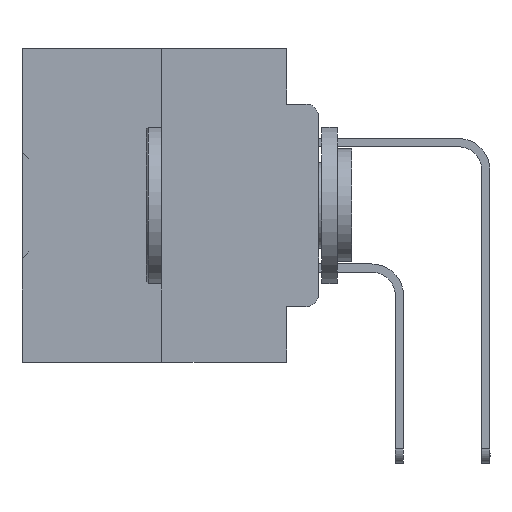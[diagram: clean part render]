
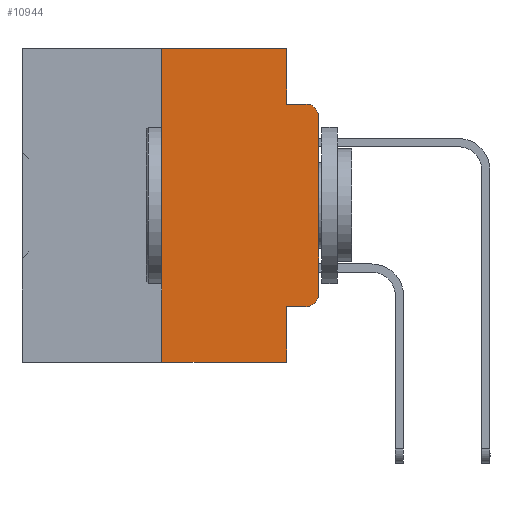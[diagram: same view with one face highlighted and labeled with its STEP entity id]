
A CAD part, left-side view. The second image highlights one B-rep face of the part: STEP entity #10944.
In plain terms, the highlighted planar face has unit normal (-1, 0, 0).
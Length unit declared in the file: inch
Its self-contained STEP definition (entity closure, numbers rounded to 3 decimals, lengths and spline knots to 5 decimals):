
#25 = DIRECTION ( 'NONE',  ( 0., -1., 0. ) ) ;
#146 = CARTESIAN_POINT ( 'NONE',  ( 0., 0., -0.1085 ) ) ;
#267 = ORIENTED_EDGE ( 'NONE', *, *, #32043, .T. ) ;
#495 = EDGE_CURVE ( 'NONE', #2584, #28971, #5270, .T. ) ;
#1047 = ORIENTED_EDGE ( 'NONE', *, *, #15151, .F. ) ;
#1120 = VERTEX_POINT ( 'NONE', #1794 ) ;
#1786 = CARTESIAN_POINT ( 'NONE',  ( 0., 0.25, -0.5 ) ) ;
#1794 = CARTESIAN_POINT ( 'NONE',  ( 0., 0.02, -0.0885 ) ) ;
#2510 = ORIENTED_EDGE ( 'NONE', *, *, #28929, .T. ) ;
#2584 = VERTEX_POINT ( 'NONE', #38696 ) ;
#2665 = CARTESIAN_POINT ( 'NONE',  ( 0., 0.473, -0.5 ) ) ;
#2685 = DIRECTION ( 'NONE',  ( -1., 0., 0. ) ) ;
#2714 = ORIENTED_EDGE ( 'NONE', *, *, #31028, .T. ) ;
#2741 = DIRECTION ( 'NONE',  ( 0., 0., -1. ) ) ;
#3422 = ORIENTED_EDGE ( 'NONE', *, *, #23063, .T. ) ;
#4181 = VERTEX_POINT ( 'NONE', #30047 ) ;
#4327 = EDGE_CURVE ( 'NONE', #29105, #31346, #19138, .T. ) ;
#4684 = CARTESIAN_POINT ( 'NONE',  ( 0., 0.25, 0. ) ) ;
#5270 = LINE ( 'NONE', #20280, #38261 ) ;
#6593 = LINE ( 'NONE', #2665, #30291 ) ;
#7724 = VERTEX_POINT ( 'NONE', #28615 ) ;
#7918 = DIRECTION ( 'NONE',  ( 0., 0., -1. ) ) ;
#8046 = AXIS2_PLACEMENT_3D ( 'NONE', #13876, #36200, #17147 ) ;
#8135 = LINE ( 'NONE', #19751, #41015 ) ;
#8181 = CARTESIAN_POINT ( 'NONE',  ( 0., 0.051, 0. ) ) ;
#8393 = CARTESIAN_POINT ( 'NONE',  ( 0., 0.051, -0.0885 ) ) ;
#10114 = DIRECTION ( 'NONE',  ( 0., 0., 1. ) ) ;
#10941 = LINE ( 'NONE', #26216, #37400 ) ;
#10944 = ADVANCED_FACE ( 'NONE', ( #22897 ), #37871, .F. ) ;
#12360 = CARTESIAN_POINT ( 'NONE',  ( 0., 0.473, 0. ) ) ;
#12381 = ORIENTED_EDGE ( 'NONE', *, *, #495, .T. ) ;
#13876 = CARTESIAN_POINT ( 'NONE',  ( 0., 0.02, -0.1085 ) ) ;
#14025 = CARTESIAN_POINT ( 'NONE',  ( 0., 0.02, -0.4115 ) ) ;
#14836 = VERTEX_POINT ( 'NONE', #1786 ) ;
#15151 = EDGE_CURVE ( 'NONE', #31346, #1120, #18486, .T. ) ;
#15672 = VERTEX_POINT ( 'NONE', #146 ) ;
#16006 = ORIENTED_EDGE ( 'NONE', *, *, #39548, .F. ) ;
#16319 = ORIENTED_EDGE ( 'NONE', *, *, #4327, .F. ) ;
#16702 = ORIENTED_EDGE ( 'NONE', *, *, #28137, .F. ) ;
#17147 = DIRECTION ( 'NONE',  ( 0., 0., -1. ) ) ;
#17576 = DIRECTION ( 'NONE',  ( 0., 0., 1. ) ) ;
#18214 = LINE ( 'NONE', #19477, #19234 ) ;
#18486 = LINE ( 'NONE', #35430, #25038 ) ;
#19138 = LINE ( 'NONE', #8181, #20149 ) ;
#19234 = VECTOR ( 'NONE', #25, 39.37008 ) ;
#19477 = CARTESIAN_POINT ( 'NONE',  ( 0., 0.473, 0. ) ) ;
#19751 = CARTESIAN_POINT ( 'NONE',  ( 0., 0., 0. ) ) ;
#20149 = VECTOR ( 'NONE', #7918, 39.37008 ) ;
#20280 = CARTESIAN_POINT ( 'NONE',  ( 0., 0.051, -0.4115 ) ) ;
#20328 = LINE ( 'NONE', #4684, #36183 ) ;
#22096 = CARTESIAN_POINT ( 'NONE',  ( 0., 0.02, -0.3915 ) ) ;
#22143 = DIRECTION ( 'NONE',  ( 1., 0., 0. ) ) ;
#22897 = FACE_OUTER_BOUND ( 'NONE', #31997, .T. ) ;
#23063 = EDGE_CURVE ( 'NONE', #28971, #7724, #39152, .T. ) ;
#24008 = VERTEX_POINT ( 'NONE', #25665 ) ;
#24355 = CARTESIAN_POINT ( 'NONE',  ( 0., 0.051, 0. ) ) ;
#24488 = ORIENTED_EDGE ( 'NONE', *, *, #38590, .F. ) ;
#25038 = VECTOR ( 'NONE', #38544, 39.37008 ) ;
#25309 = DIRECTION ( 'NONE',  ( 0., -1., 0. ) ) ;
#25323 = DIRECTION ( 'NONE',  ( 0., 0., -1. ) ) ;
#25665 = CARTESIAN_POINT ( 'NONE',  ( 0., 0.25, 0. ) ) ;
#26216 = CARTESIAN_POINT ( 'NONE',  ( 0., 0.051, 0. ) ) ;
#27052 = AXIS2_PLACEMENT_3D ( 'NONE', #22096, #2685, #25323 ) ;
#28108 = DIRECTION ( 'NONE',  ( 0., -1., 0. ) ) ;
#28137 = EDGE_CURVE ( 'NONE', #2584, #4181, #10941, .T. ) ;
#28615 = CARTESIAN_POINT ( 'NONE',  ( 0., 0., -0.3915 ) ) ;
#28929 = EDGE_CURVE ( 'NONE', #15672, #1120, #30985, .T. ) ;
#28971 = VERTEX_POINT ( 'NONE', #14025 ) ;
#29105 = VERTEX_POINT ( 'NONE', #24355 ) ;
#29441 = DIRECTION ( 'NONE',  ( 0., 0., -1. ) ) ;
#30047 = CARTESIAN_POINT ( 'NONE',  ( 0., 0.051, -0.5 ) ) ;
#30291 = VECTOR ( 'NONE', #25309, 39.37008 ) ;
#30985 = CIRCLE ( 'NONE', #8046, 0.02 ) ;
#31008 = AXIS2_PLACEMENT_3D ( 'NONE', #12360, #22143, #2741 ) ;
#31028 = EDGE_CURVE ( 'NONE', #7724, #15672, #8135, .T. ) ;
#31346 = VERTEX_POINT ( 'NONE', #8393 ) ;
#31997 = EDGE_LOOP ( 'NONE', ( #2714, #2510, #1047, #16319, #16006, #24488, #267, #16702, #12381, #3422 ) ) ;
#32043 = EDGE_CURVE ( 'NONE', #14836, #4181, #6593, .T. ) ;
#35430 = CARTESIAN_POINT ( 'NONE',  ( 0., 0.051, -0.0885 ) ) ;
#36183 = VECTOR ( 'NONE', #17576, 39.37008 ) ;
#36200 = DIRECTION ( 'NONE',  ( -1., 0., 0. ) ) ;
#37400 = VECTOR ( 'NONE', #29441, 39.37008 ) ;
#37871 = PLANE ( 'NONE',  #31008 ) ;
#38261 = VECTOR ( 'NONE', #28108, 39.37008 ) ;
#38544 = DIRECTION ( 'NONE',  ( 0., -1., 0. ) ) ;
#38590 = EDGE_CURVE ( 'NONE', #14836, #24008, #20328, .T. ) ;
#38696 = CARTESIAN_POINT ( 'NONE',  ( 0., 0.051, -0.4115 ) ) ;
#39152 = CIRCLE ( 'NONE', #27052, 0.02 ) ;
#39548 = EDGE_CURVE ( 'NONE', #24008, #29105, #18214, .T. ) ;
#41015 = VECTOR ( 'NONE', #10114, 39.37008 ) ;
